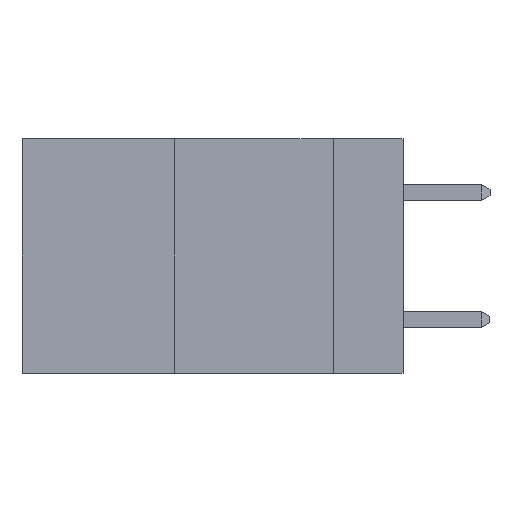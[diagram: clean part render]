
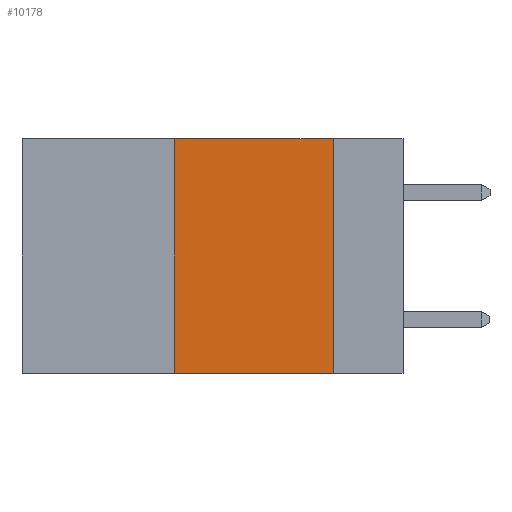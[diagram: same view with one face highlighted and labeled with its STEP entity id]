
A CAD part, left-side view. The second image highlights one B-rep face of the part: STEP entity #10178.
In plain terms, the highlighted planar face has unit normal (-1, 0, 0).
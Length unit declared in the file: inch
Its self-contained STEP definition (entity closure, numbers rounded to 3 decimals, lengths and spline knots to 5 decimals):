
#440 = VERTEX_POINT ( 'NONE', #2014 ) ;
#500 = EDGE_CURVE ( 'NONE', #5134, #440, #6908, .T. ) ;
#552 = CARTESIAN_POINT ( 'NONE',  ( 0., 0.6, 0. ) ) ;
#772 = CARTESIAN_POINT ( 'NONE',  ( 0., 0.6, -0.37 ) ) ;
#1401 = VERTEX_POINT ( 'NONE', #11617 ) ;
#1776 = VECTOR ( 'NONE', #9466, 39.37008 ) ;
#1867 = CARTESIAN_POINT ( 'NONE',  ( 0., 0.36, -0.37 ) ) ;
#1916 = ORIENTED_EDGE ( 'NONE', *, *, #6064, .F. ) ;
#2014 = CARTESIAN_POINT ( 'NONE',  ( 0., 0.36, 0. ) ) ;
#3056 = ORIENTED_EDGE ( 'NONE', *, *, #500, .F. ) ;
#3228 = VECTOR ( 'NONE', #8221, 39.37008 ) ;
#3754 = CARTESIAN_POINT ( 'NONE',  ( 0., 0.11, -0.37 ) ) ;
#4562 = PLANE ( 'NONE',  #9389 ) ;
#4853 = DIRECTION ( 'NONE',  ( 0., 0., 1. ) ) ;
#5134 = VERTEX_POINT ( 'NONE', #1867 ) ;
#5437 = LINE ( 'NONE', #552, #3228 ) ;
#5522 = DIRECTION ( 'NONE',  ( 1., 0., 0. ) ) ;
#5711 = EDGE_CURVE ( 'NONE', #1401, #9155, #8668, .T. ) ;
#6064 = EDGE_CURVE ( 'NONE', #440, #1401, #5437, .T. ) ;
#6398 = EDGE_CURVE ( 'NONE', #5134, #9155, #7411, .T. ) ;
#6433 = FACE_OUTER_BOUND ( 'NONE', #11378, .T. ) ;
#6794 = DIRECTION ( 'NONE',  ( 0., 0., -1. ) ) ;
#6908 = LINE ( 'NONE', #9038, #11141 ) ;
#7411 = LINE ( 'NONE', #772, #1776 ) ;
#8221 = DIRECTION ( 'NONE',  ( 0., -1., 0. ) ) ;
#8668 = LINE ( 'NONE', #11523, #12451 ) ;
#9038 = CARTESIAN_POINT ( 'NONE',  ( 0., 0.36, 0. ) ) ;
#9155 = VERTEX_POINT ( 'NONE', #3754 ) ;
#9389 = AXIS2_PLACEMENT_3D ( 'NONE', #12298, #5522, #9457 ) ;
#9457 = DIRECTION ( 'NONE',  ( 0., 0., -1. ) ) ;
#9466 = DIRECTION ( 'NONE',  ( 0., -1., 0. ) ) ;
#9589 = ORIENTED_EDGE ( 'NONE', *, *, #6398, .T. ) ;
#10048 = ORIENTED_EDGE ( 'NONE', *, *, #5711, .F. ) ;
#10178 = ADVANCED_FACE ( 'NONE', ( #6433 ), #4562, .F. ) ;
#11141 = VECTOR ( 'NONE', #4853, 39.37008 ) ;
#11378 = EDGE_LOOP ( 'NONE', ( #10048, #1916, #3056, #9589 ) ) ;
#11523 = CARTESIAN_POINT ( 'NONE',  ( 0., 0.11, 0. ) ) ;
#11617 = CARTESIAN_POINT ( 'NONE',  ( 0., 0.11, 0. ) ) ;
#12298 = CARTESIAN_POINT ( 'NONE',  ( 0., 0.6, 0. ) ) ;
#12451 = VECTOR ( 'NONE', #6794, 39.37008 ) ;
